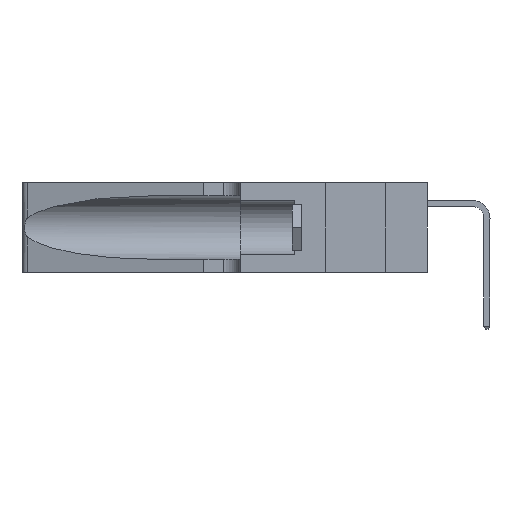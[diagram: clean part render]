
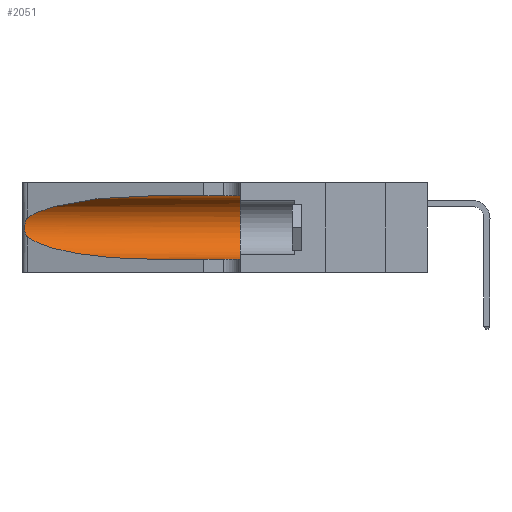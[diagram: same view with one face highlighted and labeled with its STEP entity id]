
A CAD part, left-side view. The second image highlights one B-rep face of the part: STEP entity #2051.
In plain terms, the highlighted cylindrical face has radius 3.308 mm (diameter 6.617 mm), a partial arc.
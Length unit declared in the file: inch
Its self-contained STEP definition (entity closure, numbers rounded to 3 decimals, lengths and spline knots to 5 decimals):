
#387 = CARTESIAN_POINT ( 'NONE',  ( 0.26018, 1.23835, 0.19895 ) ) ;
#1081 = AXIS2_PLACEMENT_3D ( 'NONE', #14245, #4180, #15928 ) ;
#1275 = EDGE_LOOP ( 'NONE', ( #6870, #5568, #2216, #13774, #18534, #21598 ) ) ;
#1340 = VECTOR ( 'NONE', #11661, 39.37008 ) ;
#1366 = DIRECTION ( 'NONE',  ( 0., -1., 0. ) ) ;
#1445 = CARTESIAN_POINT ( 'NONE',  ( 0.1305, 0.72297, 0.31525 ) ) ;
#1798 = CARTESIAN_POINT ( 'NONE',  ( 0.25487, 1.22718, 0.22369 ) ) ;
#1881 = LINE ( 'NONE', #19889, #1340 ) ;
#2051 = ADVANCED_FACE ( 'NONE', ( #20283 ), #19279, .F. ) ;
#2104 = CARTESIAN_POINT ( 'NONE',  ( 0.26075, 1.23896, 0.178 ) ) ;
#2216 = ORIENTED_EDGE ( 'NONE', *, *, #15284, .T. ) ;
#3731 = CARTESIAN_POINT ( 'NONE',  ( 0.1305, 0.72297, 0.05475 ) ) ;
#3772 = DIRECTION ( 'NONE',  ( 0., 0., -1. ) ) ;
#3792 = CARTESIAN_POINT ( 'NONE',  ( 0.25856, 1.23593, 0.16098 ) ) ;
#4180 = DIRECTION ( 'NONE',  ( 0., 1., 0. ) ) ;
#5349 = CARTESIAN_POINT ( 'NONE',  ( 0.25487, 1.22718, 0.14631 ) ) ;
#5479 = CARTESIAN_POINT ( 'NONE',  ( 0.25639, 1.23186, 0.15144 ) ) ;
#5568 = ORIENTED_EDGE ( 'NONE', *, *, #11028, .T. ) ;
#6538 = VERTEX_POINT ( 'NONE', #10542 ) ;
#6851 = LINE ( 'NONE', #14813, #10825 ) ;
#6870 = ORIENTED_EDGE ( 'NONE', *, *, #15059, .T. ) ;
#6948 = CARTESIAN_POINT ( 'NONE',  ( 0.25555, 1.22994, 0.2215 ) ) ;
#7098 = CARTESIAN_POINT ( 'NONE',  ( 0.25639, 1.23184, 0.21858 ) ) ;
#7175 = CARTESIAN_POINT ( 'NONE',  ( 0.25487, 1.22718, 0.14631 ) ) ;
#7826 = CARTESIAN_POINT ( 'NONE',  ( 0.25487, 1.22718, 0.14631 ) ) ;
#8220 = CARTESIAN_POINT ( 'NONE',  ( 0.25487, 1.22718, 0.22369 ) ) ;
#8319 =( BOUNDED_CURVE ( )  B_SPLINE_CURVE ( 3, ( #1445, #21433, #18223, #8220 ),
 .UNSPECIFIED., .F., .F. ) 
 B_SPLINE_CURVE_WITH_KNOTS ( ( 4, 4 ),
 ( 1.5708, 2.84003 ),
 .UNSPECIFIED. ) 
 CURVE ( )  GEOMETRIC_REPRESENTATION_ITEM ( )  RATIONAL_B_SPLINE_CURVE ( ( 1., 0.87, 0.87, 1. ) ) 
 REPRESENTATION_ITEM ( '' )  );
#8800 = CARTESIAN_POINT ( 'NONE',  ( 0.25487, 1.22718, 0.22369 ) ) ;
#9842 = AXIS2_PLACEMENT_3D ( 'NONE', #17121, #13831, #3772 ) ;
#10502 = CARTESIAN_POINT ( 'NONE',  ( 0.25854, 1.2359, 0.20912 ) ) ;
#10542 = CARTESIAN_POINT ( 'NONE',  ( 0.1305, 0.35, 0.31525 ) ) ;
#10767 = EDGE_CURVE ( 'NONE', #18587, #6538, #6851, .T. ) ;
#10825 = VECTOR ( 'NONE', #1366, 39.37008 ) ;
#11028 = EDGE_CURVE ( 'NONE', #15832, #19328, #17323, .T. ) ;
#11661 = DIRECTION ( 'NONE',  ( 0., -1., 0. ) ) ;
#11975 = EDGE_CURVE ( 'NONE', #13840, #18801, #1881, .T. ) ;
#12194 = CARTESIAN_POINT ( 'NONE',  ( 0.26075, 1.23896, 0.19203 ) ) ;
#13208 = CARTESIAN_POINT ( 'NONE',  ( 0.1305, 0.72297, 0.05475 ) ) ;
#13305 = CARTESIAN_POINT ( 'NONE',  ( 0.1305, 0.72297, 0.31525 ) ) ;
#13774 = ORIENTED_EDGE ( 'NONE', *, *, #11975, .T. ) ;
#13790 = CARTESIAN_POINT ( 'NONE',  ( 0.18966, 0.96281, 0.05475 ) ) ;
#13831 = DIRECTION ( 'NONE',  ( 0., -1., 0. ) ) ;
#13840 = VERTEX_POINT ( 'NONE', #13208 ) ;
#13849 = CARTESIAN_POINT ( 'NONE',  ( 0.26017, 1.23833, 0.17102 ) ) ;
#14245 = CARTESIAN_POINT ( 'NONE',  ( 0.1305, 0.35, 0.185 ) ) ;
#14813 = CARTESIAN_POINT ( 'NONE',  ( 0.1305, 1.61858, 0.31525 ) ) ;
#15059 = EDGE_CURVE ( 'NONE', #18587, #15832, #8319, .T. ) ;
#15284 = EDGE_CURVE ( 'NONE', #19328, #13840, #17975, .T. ) ;
#15531 = CARTESIAN_POINT ( 'NONE',  ( 0.25789, 1.23486, 0.15765 ) ) ;
#15832 = VERTEX_POINT ( 'NONE', #1798 ) ;
#15928 = DIRECTION ( 'NONE',  ( 0., 0., 1. ) ) ;
#17121 = CARTESIAN_POINT ( 'NONE',  ( 0.1305, 1.61858, 0.185 ) ) ;
#17207 = CARTESIAN_POINT ( 'NONE',  ( 0.25555, 1.22993, 0.14849 ) ) ;
#17323 = B_SPLINE_CURVE_WITH_KNOTS ( 'NONE', 3,
 ( #8800, #6948, #7098, #20408, #10502, #387, #12194, #2104, #13849, #3792, #15531, #5479, #17207, #7175 ),
 .UNSPECIFIED., .F., .F.,
 ( 4, 2, 2, 2, 2, 2, 4 ),
 ( 0., 0.00027, 0.00053, 0.00107, 0.0016, 0.00187, 0.00214 ),
 .UNSPECIFIED. ) ;
#17975 =( BOUNDED_CURVE ( )  B_SPLINE_CURVE ( 3, ( #5349, #18719, #13790, #3731 ),
 .UNSPECIFIED., .F., .T. ) 
 B_SPLINE_CURVE_WITH_KNOTS ( ( 4, 4 ),
 ( 3.44316, 4.71239 ),
 .UNSPECIFIED. ) 
 CURVE ( )  GEOMETRIC_REPRESENTATION_ITEM ( )  RATIONAL_B_SPLINE_CURVE ( ( 1., 0.87, 0.87, 1. ) ) 
 REPRESENTATION_ITEM ( '' )  );
#18223 = CARTESIAN_POINT ( 'NONE',  ( 0.2373, 1.15595, 0.28018 ) ) ;
#18534 = ORIENTED_EDGE ( 'NONE', *, *, #20370, .F. ) ;
#18587 = VERTEX_POINT ( 'NONE', #13305 ) ;
#18719 = CARTESIAN_POINT ( 'NONE',  ( 0.2373, 1.15595, 0.08982 ) ) ;
#18801 = VERTEX_POINT ( 'NONE', #20574 ) ;
#18898 = CIRCLE ( 'NONE', #1081, 0.13025 ) ;
#19279 = CYLINDRICAL_SURFACE ( 'NONE', #9842, 0.13025 ) ;
#19328 = VERTEX_POINT ( 'NONE', #7826 ) ;
#19889 = CARTESIAN_POINT ( 'NONE',  ( 0.1305, 1.61858, 0.05475 ) ) ;
#20283 = FACE_OUTER_BOUND ( 'NONE', #1275, .T. ) ;
#20370 = EDGE_CURVE ( 'NONE', #6538, #18801, #18898, .T. ) ;
#20408 = CARTESIAN_POINT ( 'NONE',  ( 0.25787, 1.23484, 0.2124 ) ) ;
#20574 = CARTESIAN_POINT ( 'NONE',  ( 0.1305, 0.35, 0.05475 ) ) ;
#21433 = CARTESIAN_POINT ( 'NONE',  ( 0.18966, 0.96281, 0.31525 ) ) ;
#21598 = ORIENTED_EDGE ( 'NONE', *, *, #10767, .F. ) ;
